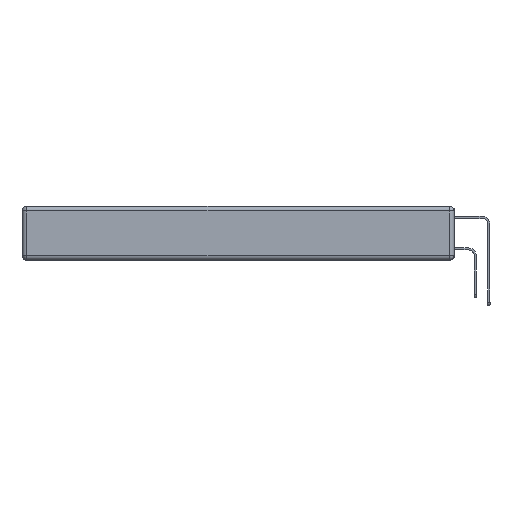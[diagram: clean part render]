
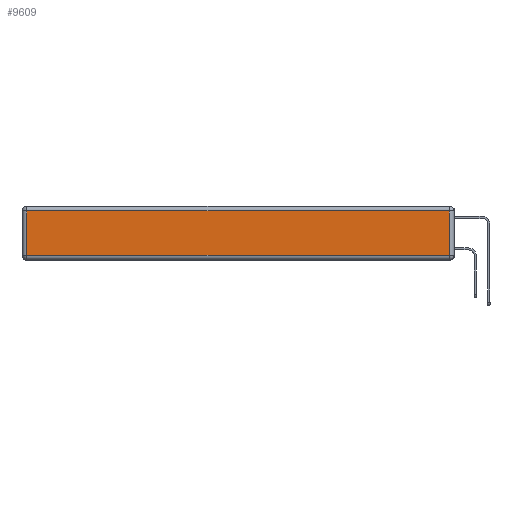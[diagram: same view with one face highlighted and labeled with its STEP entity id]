
A CAD part, left-side view. The second image highlights one B-rep face of the part: STEP entity #9609.
In plain terms, the highlighted planar face has unit normal (-1, 0, 0).
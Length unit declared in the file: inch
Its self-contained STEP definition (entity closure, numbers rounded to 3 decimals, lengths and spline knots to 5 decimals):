
#1811 = LINE ( 'NONE', #23191, #17241 ) ;
#2460 = ORIENTED_EDGE ( 'NONE', *, *, #27624, .T. ) ;
#3304 = EDGE_CURVE ( 'NONE', #23868, #11425, #9088, .T. ) ;
#6062 = EDGE_CURVE ( 'NONE', #25598, #23868, #12991, .T. ) ;
#6103 = DIRECTION ( 'NONE',  ( 0., -1., 0. ) ) ;
#6830 = VECTOR ( 'NONE', #26501, 39.37008 ) ;
#8676 = CARTESIAN_POINT ( 'NONE',  ( 0., 0.03, -0.313 ) ) ;
#9088 = LINE ( 'NONE', #11386, #6830 ) ;
#9321 = LINE ( 'NONE', #18282, #9420 ) ;
#9420 = VECTOR ( 'NONE', #15823, 39.37008 ) ;
#9609 = ADVANCED_FACE ( 'NONE', ( #17826 ), #22341, .T. ) ;
#11386 = CARTESIAN_POINT ( 'NONE',  ( 0., 0.03, -0.343 ) ) ;
#11425 = VERTEX_POINT ( 'NONE', #18235 ) ;
#12991 = LINE ( 'NONE', #23604, #21750 ) ;
#13607 = VERTEX_POINT ( 'NONE', #25086 ) ;
#14439 = ORIENTED_EDGE ( 'NONE', *, *, #26432, .T. ) ;
#15823 = DIRECTION ( 'NONE',  ( 0., 1., 0. ) ) ;
#16701 = AXIS2_PLACEMENT_3D ( 'NONE', #26700, #19446, #28317 ) ;
#17241 = VECTOR ( 'NONE', #23479, 39.37008 ) ;
#17826 = FACE_OUTER_BOUND ( 'NONE', #20143, .T. ) ;
#18235 = CARTESIAN_POINT ( 'NONE',  ( 0., 0.03, -0.03 ) ) ;
#18282 = CARTESIAN_POINT ( 'NONE',  ( 0., 2.75, -0.03 ) ) ;
#19446 = DIRECTION ( 'NONE',  ( -1., 0., 0. ) ) ;
#20143 = EDGE_LOOP ( 'NONE', ( #21197, #22086, #2460, #14439 ) ) ;
#21197 = ORIENTED_EDGE ( 'NONE', *, *, #6062, .T. ) ;
#21750 = VECTOR ( 'NONE', #6103, 39.37008 ) ;
#22086 = ORIENTED_EDGE ( 'NONE', *, *, #3304, .T. ) ;
#22341 = PLANE ( 'NONE',  #16701 ) ;
#22426 = CARTESIAN_POINT ( 'NONE',  ( 0., 2.72, -0.313 ) ) ;
#23191 = CARTESIAN_POINT ( 'NONE',  ( 0., 2.72, -0.343 ) ) ;
#23479 = DIRECTION ( 'NONE',  ( 0., 0., -1. ) ) ;
#23604 = CARTESIAN_POINT ( 'NONE',  ( 0., 0., -0.313 ) ) ;
#23868 = VERTEX_POINT ( 'NONE', #8676 ) ;
#25086 = CARTESIAN_POINT ( 'NONE',  ( 0., 2.72, -0.03 ) ) ;
#25598 = VERTEX_POINT ( 'NONE', #22426 ) ;
#26432 = EDGE_CURVE ( 'NONE', #13607, #25598, #1811, .T. ) ;
#26501 = DIRECTION ( 'NONE',  ( 0., 0., 1. ) ) ;
#26700 = CARTESIAN_POINT ( 'NONE',  ( 0., 0., -0.343 ) ) ;
#27624 = EDGE_CURVE ( 'NONE', #11425, #13607, #9321, .T. ) ;
#28317 = DIRECTION ( 'NONE',  ( 0., 0., 1. ) ) ;
